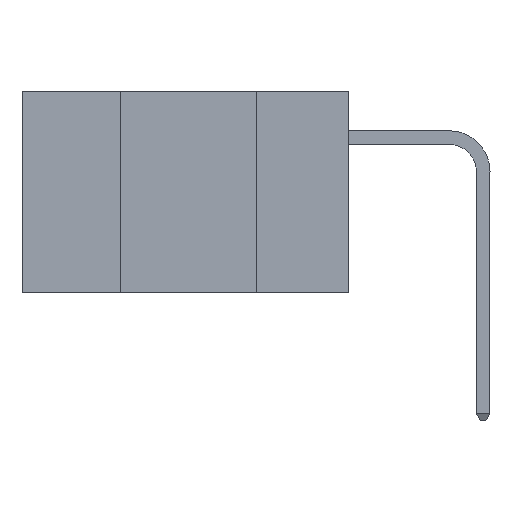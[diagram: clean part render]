
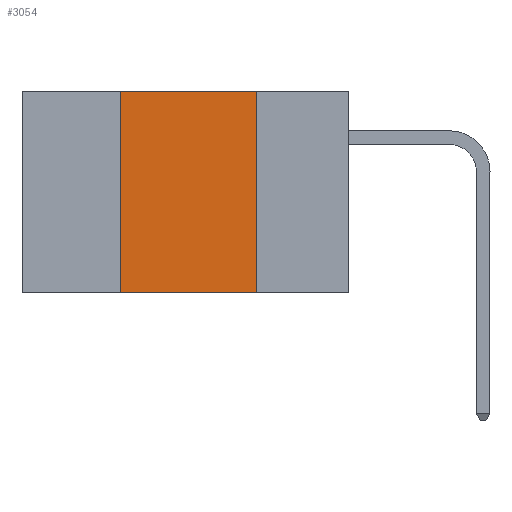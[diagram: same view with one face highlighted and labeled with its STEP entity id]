
A CAD part, left-side view. The second image highlights one B-rep face of the part: STEP entity #3054.
In plain terms, the highlighted planar face has unit normal (-1, 0, 0).
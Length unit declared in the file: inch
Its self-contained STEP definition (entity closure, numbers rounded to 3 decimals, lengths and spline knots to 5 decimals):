
#584 = LINE ( 'NONE', #19137, #8045 ) ;
#1751 = PLANE ( 'NONE',  #18819 ) ;
#2532 = EDGE_CURVE ( 'NONE', #5916, #22534, #9673, .T. ) ;
#3054 = ADVANCED_FACE ( 'NONE', ( #3201 ), #1751, .F. ) ;
#3201 = FACE_OUTER_BOUND ( 'NONE', #22531, .T. ) ;
#3605 = EDGE_CURVE ( 'NONE', #16344, #22534, #11487, .T. ) ;
#3684 = CARTESIAN_POINT ( 'NONE',  ( 0., 0.6, 0. ) ) ;
#4180 = ORIENTED_EDGE ( 'NONE', *, *, #3605, .T. ) ;
#4690 = ORIENTED_EDGE ( 'NONE', *, *, #10429, .F. ) ;
#5499 = CARTESIAN_POINT ( 'NONE',  ( 0., 0.6, -0.37 ) ) ;
#5834 = DIRECTION ( 'NONE',  ( 1., 0., 0. ) ) ;
#5916 = VERTEX_POINT ( 'NONE', #6956 ) ;
#6956 = CARTESIAN_POINT ( 'NONE',  ( 0., 0.17, 0. ) ) ;
#8045 = VECTOR ( 'NONE', #11466, 39.37008 ) ;
#9673 = LINE ( 'NONE', #13610, #23278 ) ;
#10429 = EDGE_CURVE ( 'NONE', #18925, #5916, #584, .T. ) ;
#11466 = DIRECTION ( 'NONE',  ( 0., -1., 0. ) ) ;
#11487 = LINE ( 'NONE', #5499, #14871 ) ;
#11998 = DIRECTION ( 'NONE',  ( 0., 0., 1. ) ) ;
#13610 = CARTESIAN_POINT ( 'NONE',  ( 0., 0.17, 0. ) ) ;
#14387 = CARTESIAN_POINT ( 'NONE',  ( 0., 0.42, -0.37 ) ) ;
#14871 = VECTOR ( 'NONE', #18469, 39.37008 ) ;
#15344 = DIRECTION ( 'NONE',  ( 0., 0., -1. ) ) ;
#15559 = DIRECTION ( 'NONE',  ( 0., 0., -1. ) ) ;
#15989 = LINE ( 'NONE', #22123, #24369 ) ;
#16311 = ORIENTED_EDGE ( 'NONE', *, *, #2532, .F. ) ;
#16344 = VERTEX_POINT ( 'NONE', #14387 ) ;
#18469 = DIRECTION ( 'NONE',  ( 0., -1., 0. ) ) ;
#18620 = EDGE_CURVE ( 'NONE', #16344, #18925, #15989, .T. ) ;
#18819 = AXIS2_PLACEMENT_3D ( 'NONE', #3684, #5834, #15559 ) ;
#18925 = VERTEX_POINT ( 'NONE', #19070 ) ;
#19070 = CARTESIAN_POINT ( 'NONE',  ( 0., 0.42, 0. ) ) ;
#19137 = CARTESIAN_POINT ( 'NONE',  ( 0., 0.6, 0. ) ) ;
#22123 = CARTESIAN_POINT ( 'NONE',  ( 0., 0.42, 0. ) ) ;
#22531 = EDGE_LOOP ( 'NONE', ( #16311, #4690, #22845, #4180 ) ) ;
#22534 = VERTEX_POINT ( 'NONE', #24429 ) ;
#22845 = ORIENTED_EDGE ( 'NONE', *, *, #18620, .F. ) ;
#23278 = VECTOR ( 'NONE', #15344, 39.37008 ) ;
#24369 = VECTOR ( 'NONE', #11998, 39.37008 ) ;
#24429 = CARTESIAN_POINT ( 'NONE',  ( 0., 0.17, -0.37 ) ) ;
